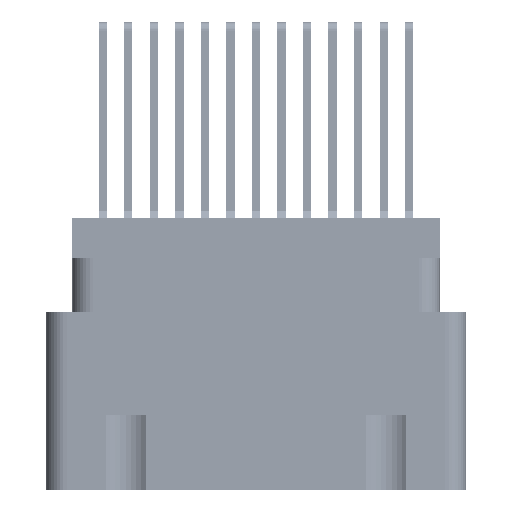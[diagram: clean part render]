
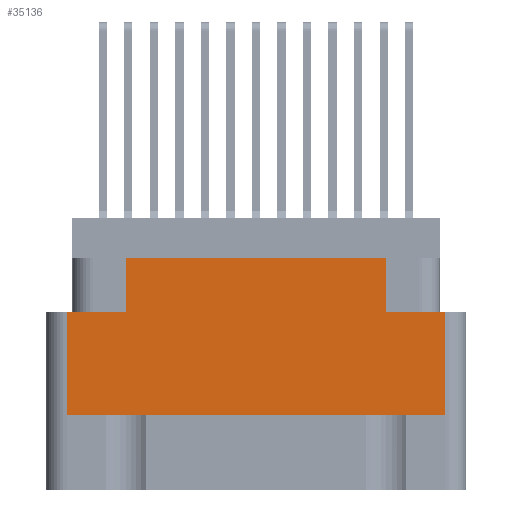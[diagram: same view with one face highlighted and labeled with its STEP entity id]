
A CAD part, left-side view. The second image highlights one B-rep face of the part: STEP entity #35136.
In plain terms, the highlighted planar face has unit normal (-1, 0, 0).
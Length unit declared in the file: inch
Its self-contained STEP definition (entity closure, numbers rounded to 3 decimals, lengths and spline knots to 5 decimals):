
#163 = DIRECTION ( 'NONE',  ( 0., 0., 1. ) ) ;
#2753 = CARTESIAN_POINT ( 'NONE',  ( -1.359, 0., -0.274 ) ) ;
#3114 = LINE ( 'NONE', #26227, #39269 ) ;
#3875 = VERTEX_POINT ( 'NONE', #50537 ) ;
#5211 = VECTOR ( 'NONE', #42310, 39.37008 ) ;
#5299 = EDGE_CURVE ( 'NONE', #46852, #59474, #36241, .T. ) ;
#5474 = CARTESIAN_POINT ( 'NONE',  ( -1.359, -0.555, -0.274 ) ) ;
#8018 = CARTESIAN_POINT ( 'NONE',  ( -1.359, 0., -0.274 ) ) ;
#8515 = LINE ( 'NONE', #62717, #5211 ) ;
#9691 = VERTEX_POINT ( 'NONE', #5474 ) ;
#11941 = ORIENTED_EDGE ( 'NONE', *, *, #28854, .F. ) ;
#12089 = CARTESIAN_POINT ( 'NONE',  ( -1.359, 0.3825, -0.274 ) ) ;
#13751 = DIRECTION ( 'NONE',  ( 0., -1., 0. ) ) ;
#14257 = ORIENTED_EDGE ( 'NONE', *, *, #15320, .T. ) ;
#15320 = EDGE_CURVE ( 'NONE', #3875, #29817, #23485, .T. ) ;
#16542 = FACE_OUTER_BOUND ( 'NONE', #51951, .T. ) ;
#17461 = LINE ( 'NONE', #8018, #66671 ) ;
#18357 = VERTEX_POINT ( 'NONE', #50145 ) ;
#21388 = VERTEX_POINT ( 'NONE', #30046 ) ;
#21683 = LINE ( 'NONE', #26936, #51151 ) ;
#23485 = LINE ( 'NONE', #58847, #50672 ) ;
#26023 = CARTESIAN_POINT ( 'NONE',  ( -1.359, -0.617, -0.798 ) ) ;
#26227 = CARTESIAN_POINT ( 'NONE',  ( -1.359, 0.617, -0.117 ) ) ;
#26478 = DIRECTION ( 'NONE',  ( 0., 0., 1. ) ) ;
#26552 = LINE ( 'NONE', #50501, #37243 ) ;
#26683 = DIRECTION ( 'NONE',  ( 0., -1., 0. ) ) ;
#26936 = CARTESIAN_POINT ( 'NONE',  ( -1.359, -0.3825, -0.274 ) ) ;
#27322 = DIRECTION ( 'NONE',  ( 0., 0., -1. ) ) ;
#28854 = EDGE_CURVE ( 'NONE', #59474, #18357, #3114, .T. ) ;
#29817 = VERTEX_POINT ( 'NONE', #67702 ) ;
#30046 = CARTESIAN_POINT ( 'NONE',  ( -1.359, -0.3825, -0.274 ) ) ;
#30849 = PLANE ( 'NONE',  #32155 ) ;
#31222 = ORIENTED_EDGE ( 'NONE', *, *, #65565, .F. ) ;
#31321 = DIRECTION ( 'NONE',  ( -1., 0., 0. ) ) ;
#32155 = AXIS2_PLACEMENT_3D ( 'NONE', #26023, #31321, #163 ) ;
#32318 = ORIENTED_EDGE ( 'NONE', *, *, #47234, .T. ) ;
#35136 = ADVANCED_FACE ( 'NONE', ( #16542 ), #30849, .T. ) ;
#36241 = LINE ( 'NONE', #55908, #57644 ) ;
#37243 = VECTOR ( 'NONE', #13751, 39.37008 ) ;
#39269 = VECTOR ( 'NONE', #26683, 39.37008 ) ;
#41715 = ORIENTED_EDGE ( 'NONE', *, *, #48635, .T. ) ;
#42310 = DIRECTION ( 'NONE',  ( 0., 0., 1. ) ) ;
#42897 = CARTESIAN_POINT ( 'NONE',  ( -1.359, -0.555, -0.578 ) ) ;
#44157 = ORIENTED_EDGE ( 'NONE', *, *, #58193, .T. ) ;
#46721 = ORIENTED_EDGE ( 'NONE', *, *, #66556, .F. ) ;
#46852 = VERTEX_POINT ( 'NONE', #12089 ) ;
#47234 = EDGE_CURVE ( 'NONE', #21388, #18357, #21683, .T. ) ;
#48635 = EDGE_CURVE ( 'NONE', #29817, #61796, #26552, .T. ) ;
#50145 = CARTESIAN_POINT ( 'NONE',  ( -1.359, -0.3825, -0.117 ) ) ;
#50501 = CARTESIAN_POINT ( 'NONE',  ( -1.359, 0., -0.578 ) ) ;
#50537 = CARTESIAN_POINT ( 'NONE',  ( -1.359, 0.555, -0.274 ) ) ;
#50672 = VECTOR ( 'NONE', #27322, 39.37008 ) ;
#51151 = VECTOR ( 'NONE', #26478, 39.37008 ) ;
#51951 = EDGE_LOOP ( 'NONE', ( #31222, #14257, #41715, #44157, #46721, #32318, #11941, #53045 ) ) ;
#53045 = ORIENTED_EDGE ( 'NONE', *, *, #5299, .F. ) ;
#53091 = CARTESIAN_POINT ( 'NONE',  ( -1.359, 0.3825, -0.117 ) ) ;
#55908 = CARTESIAN_POINT ( 'NONE',  ( -1.359, 0.3825, -0.274 ) ) ;
#57644 = VECTOR ( 'NONE', #61598, 39.37008 ) ;
#58193 = EDGE_CURVE ( 'NONE', #61796, #9691, #8515, .T. ) ;
#58847 = CARTESIAN_POINT ( 'NONE',  ( -1.359, 0.555, -0.798 ) ) ;
#59474 = VERTEX_POINT ( 'NONE', #53091 ) ;
#61188 = VECTOR ( 'NONE', #65808, 39.37008 ) ;
#61598 = DIRECTION ( 'NONE',  ( 0., 0., 1. ) ) ;
#61796 = VERTEX_POINT ( 'NONE', #42897 ) ;
#62717 = CARTESIAN_POINT ( 'NONE',  ( -1.359, -0.555, -0.798 ) ) ;
#63596 = LINE ( 'NONE', #2753, #61188 ) ;
#65565 = EDGE_CURVE ( 'NONE', #3875, #46852, #63596, .T. ) ;
#65808 = DIRECTION ( 'NONE',  ( 0., -1., 0. ) ) ;
#66234 = DIRECTION ( 'NONE',  ( 0., -1., 0. ) ) ;
#66556 = EDGE_CURVE ( 'NONE', #21388, #9691, #17461, .T. ) ;
#66671 = VECTOR ( 'NONE', #66234, 39.37008 ) ;
#67702 = CARTESIAN_POINT ( 'NONE',  ( -1.359, 0.555, -0.578 ) ) ;
